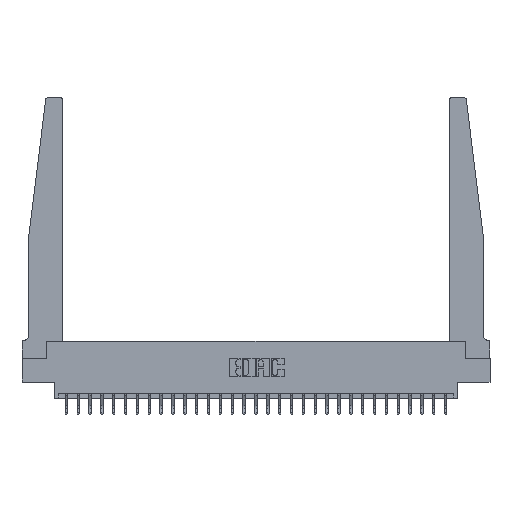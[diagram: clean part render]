
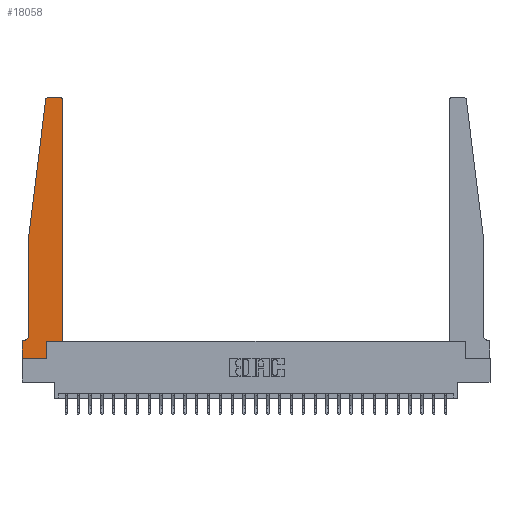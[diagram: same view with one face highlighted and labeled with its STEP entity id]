
A CAD part, top view. The second image highlights one B-rep face of the part: STEP entity #18058.
In plain terms, the highlighted planar face has unit normal (0, 0, 1).
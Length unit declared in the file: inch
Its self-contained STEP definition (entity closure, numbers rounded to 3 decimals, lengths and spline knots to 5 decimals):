
#94 = EDGE_CURVE ( 'NONE', #17533, #21609, #1661, .T. ) ;
#211 = LINE ( 'NONE', #19964, #15068 ) ;
#486 = VERTEX_POINT ( 'NONE', #12643 ) ;
#611 = LINE ( 'NONE', #3167, #12998 ) ;
#1375 = DIRECTION ( 'NONE',  ( 0., 0., 1. ) ) ;
#1379 = VERTEX_POINT ( 'NONE', #2944 ) ;
#1468 = LINE ( 'NONE', #10199, #11480 ) ;
#1661 = CIRCLE ( 'NONE', #8976, 0.05 ) ;
#1673 = CARTESIAN_POINT ( 'NONE',  ( 0.015, 0.2375, 0.37 ) ) ;
#1821 = EDGE_CURVE ( 'NONE', #2928, #486, #24411, .T. ) ;
#2097 = DIRECTION ( 'NONE',  ( -1., 0., 0. ) ) ;
#2598 = CARTESIAN_POINT ( 'NONE',  ( 0.425, 2.72, 0.37 ) ) ;
#2751 = ORIENTED_EDGE ( 'NONE', *, *, #3650, .T. ) ;
#2810 = CARTESIAN_POINT ( 'NONE',  ( 0., 0.1875, 0.37 ) ) ;
#2928 = VERTEX_POINT ( 'NONE', #22994 ) ;
#2944 = CARTESIAN_POINT ( 'NONE',  ( 0.27653, 2.75, 0.37 ) ) ;
#3167 = CARTESIAN_POINT ( 'NONE',  ( 0.065, 0.1875, 0.37 ) ) ;
#3507 = CARTESIAN_POINT ( 'NONE',  ( 0.2605, 0., 0.37 ) ) ;
#3650 = EDGE_CURVE ( 'NONE', #21043, #24631, #9616, .T. ) ;
#3784 = ORIENTED_EDGE ( 'NONE', *, *, #10449, .T. ) ;
#3857 = AXIS2_PLACEMENT_3D ( 'NONE', #15150, #4285, #23909 ) ;
#3962 = ORIENTED_EDGE ( 'NONE', *, *, #26503, .T. ) ;
#4098 = ORIENTED_EDGE ( 'NONE', *, *, #7874, .T. ) ;
#4285 = DIRECTION ( 'NONE',  ( 0., 0., 1. ) ) ;
#4299 = CARTESIAN_POINT ( 'NONE',  ( 0.24675, 2.72367, 0.37 ) ) ;
#4304 = VERTEX_POINT ( 'NONE', #25497 ) ;
#4775 = DIRECTION ( 'NONE',  ( 0., -1., 0. ) ) ;
#4904 = DIRECTION ( 'NONE',  ( -1., 0., 0. ) ) ;
#4981 = EDGE_CURVE ( 'NONE', #21609, #2928, #611, .T. ) ;
#5205 = VECTOR ( 'NONE', #14563, 39.37008 ) ;
#5362 = ORIENTED_EDGE ( 'NONE', *, *, #1821, .T. ) ;
#6559 = VECTOR ( 'NONE', #20179, 39.37008 ) ;
#7159 = CARTESIAN_POINT ( 'NONE',  ( 0., 0., 0.37 ) ) ;
#7641 = DIRECTION ( 'NONE',  ( 1., 0., 0. ) ) ;
#7874 = EDGE_CURVE ( 'NONE', #24631, #27738, #9077, .T. ) ;
#8165 = AXIS2_PLACEMENT_3D ( 'NONE', #24014, #25143, #26888 ) ;
#8233 = VECTOR ( 'NONE', #12973, 39.37008 ) ;
#8926 = ORIENTED_EDGE ( 'NONE', *, *, #16399, .T. ) ;
#8940 = DIRECTION ( 'NONE',  ( -1., 0., 0. ) ) ;
#8976 = AXIS2_PLACEMENT_3D ( 'NONE', #1673, #17137, #2097 ) ;
#9077 = CIRCLE ( 'NONE', #8165, 0.03 ) ;
#9468 = CARTESIAN_POINT ( 'NONE',  ( 0.2605, 0.18, 0.37 ) ) ;
#9616 = LINE ( 'NONE', #11341, #11442 ) ;
#9658 = EDGE_CURVE ( 'NONE', #27738, #1379, #211, .T. ) ;
#10047 = ORIENTED_EDGE ( 'NONE', *, *, #9658, .T. ) ;
#10199 = CARTESIAN_POINT ( 'NONE',  ( 0.425, 0.18, 0.37 ) ) ;
#10225 = CARTESIAN_POINT ( 'NONE',  ( 0.015, 0.1875, 0.37 ) ) ;
#10418 = LINE ( 'NONE', #16734, #5205 ) ;
#10449 = EDGE_CURVE ( 'NONE', #17688, #17533, #10838, .T. ) ;
#10838 = LINE ( 'NONE', #23873, #8233 ) ;
#11341 = CARTESIAN_POINT ( 'NONE',  ( 0.425, 0.18, 0.37 ) ) ;
#11442 = VECTOR ( 'NONE', #26837, 39.37008 ) ;
#11480 = VECTOR ( 'NONE', #7641, 39.37008 ) ;
#12643 = CARTESIAN_POINT ( 'NONE',  ( 0., 0., 0.37 ) ) ;
#12973 = DIRECTION ( 'NONE',  ( 0., -1., 0. ) ) ;
#12998 = VECTOR ( 'NONE', #4904, 39.37008 ) ;
#13007 = EDGE_CURVE ( 'NONE', #4304, #21043, #1468, .T. ) ;
#14161 = VERTEX_POINT ( 'NONE', #3507 ) ;
#14563 = DIRECTION ( 'NONE',  ( -0.122, -0.992, 0. ) ) ;
#14826 = ORIENTED_EDGE ( 'NONE', *, *, #23443, .T. ) ;
#15068 = VECTOR ( 'NONE', #8940, 39.37008 ) ;
#15150 = CARTESIAN_POINT ( 'NONE',  ( 0.27653, 2.72, 0.37 ) ) ;
#15188 = VECTOR ( 'NONE', #15909, 39.37008 ) ;
#15798 = CARTESIAN_POINT ( 'NONE',  ( 0., 0., 0.37 ) ) ;
#15909 = DIRECTION ( 'NONE',  ( 0., 1., 0. ) ) ;
#16399 = EDGE_CURVE ( 'NONE', #27435, #17688, #10418, .T. ) ;
#16414 = FACE_OUTER_BOUND ( 'NONE', #18709, .T. ) ;
#16734 = CARTESIAN_POINT ( 'NONE',  ( 0.065, 1.25, 0.37 ) ) ;
#16789 = ORIENTED_EDGE ( 'NONE', *, *, #18913, .T. ) ;
#17137 = DIRECTION ( 'NONE',  ( 0., 0., -1. ) ) ;
#17533 = VERTEX_POINT ( 'NONE', #18460 ) ;
#17688 = VERTEX_POINT ( 'NONE', #21589 ) ;
#18058 = ADVANCED_FACE ( 'NONE', ( #16414 ), #22434, .T. ) ;
#18159 = CARTESIAN_POINT ( 'NONE',  ( 0.425, 0.18, 0.37 ) ) ;
#18460 = CARTESIAN_POINT ( 'NONE',  ( 0.065, 0.2375, 0.37 ) ) ;
#18709 = EDGE_LOOP ( 'NONE', ( #10047, #16789, #8926, #3784, #25330, #20070, #5362, #3962, #14826, #25888, #2751, #4098 ) ) ;
#18843 = DIRECTION ( 'NONE',  ( 1., 0., 0. ) ) ;
#18913 = EDGE_CURVE ( 'NONE', #1379, #27435, #19421, .T. ) ;
#19421 = CIRCLE ( 'NONE', #3857, 0.03 ) ;
#19964 = CARTESIAN_POINT ( 'NONE',  ( 0.25, 2.75, 0.37 ) ) ;
#20070 = ORIENTED_EDGE ( 'NONE', *, *, #4981, .T. ) ;
#20179 = DIRECTION ( 'NONE',  ( 1., 0., 0. ) ) ;
#21043 = VERTEX_POINT ( 'NONE', #18159 ) ;
#21589 = CARTESIAN_POINT ( 'NONE',  ( 0.065, 1.25, 0.37 ) ) ;
#21609 = VERTEX_POINT ( 'NONE', #10225 ) ;
#22434 = PLANE ( 'NONE',  #24870 ) ;
#22994 = CARTESIAN_POINT ( 'NONE',  ( 0., 0.1875, 0.37 ) ) ;
#23443 = EDGE_CURVE ( 'NONE', #14161, #4304, #26541, .T. ) ;
#23873 = CARTESIAN_POINT ( 'NONE',  ( 0.065, 1.25, 0.37 ) ) ;
#23909 = DIRECTION ( 'NONE',  ( 1., 0., 0. ) ) ;
#24014 = CARTESIAN_POINT ( 'NONE',  ( 0.395, 2.72, 0.37 ) ) ;
#24411 = LINE ( 'NONE', #15798, #25866 ) ;
#24431 = CARTESIAN_POINT ( 'NONE',  ( 0.395, 2.75, 0.37 ) ) ;
#24631 = VERTEX_POINT ( 'NONE', #2598 ) ;
#24870 = AXIS2_PLACEMENT_3D ( 'NONE', #2810, #1375, #18843 ) ;
#25143 = DIRECTION ( 'NONE',  ( 0., 0., 1. ) ) ;
#25330 = ORIENTED_EDGE ( 'NONE', *, *, #94, .T. ) ;
#25497 = CARTESIAN_POINT ( 'NONE',  ( 0.2605, 0.18, 0.37 ) ) ;
#25866 = VECTOR ( 'NONE', #4775, 39.37008 ) ;
#25888 = ORIENTED_EDGE ( 'NONE', *, *, #13007, .T. ) ;
#26503 = EDGE_CURVE ( 'NONE', #486, #14161, #26797, .T. ) ;
#26541 = LINE ( 'NONE', #9468, #15188 ) ;
#26797 = LINE ( 'NONE', #7159, #6559 ) ;
#26837 = DIRECTION ( 'NONE',  ( 0., 1., 0. ) ) ;
#26888 = DIRECTION ( 'NONE',  ( 1., 0., 0. ) ) ;
#27435 = VERTEX_POINT ( 'NONE', #4299 ) ;
#27738 = VERTEX_POINT ( 'NONE', #24431 ) ;
